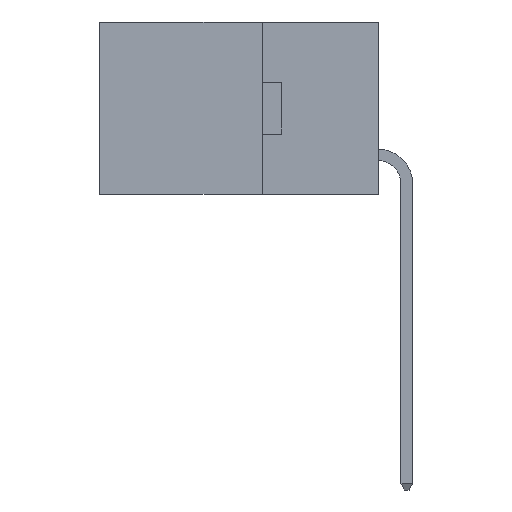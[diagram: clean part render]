
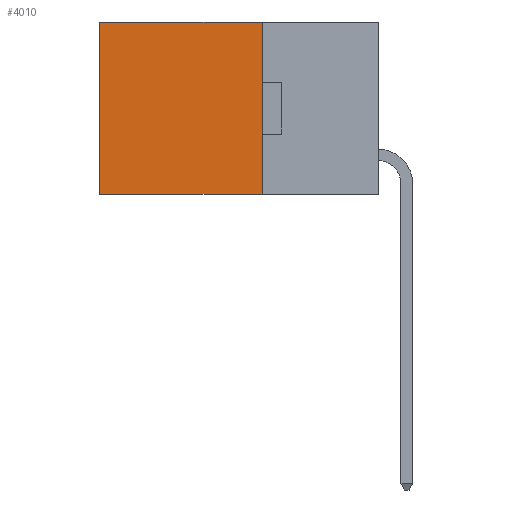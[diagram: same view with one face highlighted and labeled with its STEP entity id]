
A CAD part, left-side view. The second image highlights one B-rep face of the part: STEP entity #4010.
In plain terms, the highlighted planar face has unit normal (-1, 0, 0).
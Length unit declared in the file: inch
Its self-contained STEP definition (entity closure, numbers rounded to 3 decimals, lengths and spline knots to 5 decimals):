
#916 = CARTESIAN_POINT ( 'NONE',  ( 0.2615, 0.25, -0.37 ) ) ;
#2345 = LINE ( 'NONE', #15793, #16446 ) ;
#2472 = EDGE_CURVE ( 'NONE', #17665, #14523, #2345, .T. ) ;
#2713 = EDGE_CURVE ( 'NONE', #25090, #12654, #26334, .T. ) ;
#4010 = ADVANCED_FACE ( 'NONE', ( #21203 ), #24283, .F. ) ;
#4569 = CARTESIAN_POINT ( 'NONE',  ( 0.2615, 0.6, 0. ) ) ;
#4777 = EDGE_LOOP ( 'NONE', ( #15254, #18276, #24194, #24039 ) ) ;
#4930 = VECTOR ( 'NONE', #5220, 39.37008 ) ;
#5220 = DIRECTION ( 'NONE',  ( 0., 0., -1. ) ) ;
#6116 = CARTESIAN_POINT ( 'NONE',  ( 0.2615, 0.25, 0. ) ) ;
#8182 = CARTESIAN_POINT ( 'NONE',  ( 0.2615, 0.6, -0.37 ) ) ;
#8214 = EDGE_CURVE ( 'NONE', #17665, #25090, #16729, .T. ) ;
#10292 = DIRECTION ( 'NONE',  ( 0., 0., -1. ) ) ;
#12654 = VERTEX_POINT ( 'NONE', #14967 ) ;
#12839 = DIRECTION ( 'NONE',  ( 0., 1., 0. ) ) ;
#13164 = LINE ( 'NONE', #8182, #23462 ) ;
#14523 = VERTEX_POINT ( 'NONE', #4569 ) ;
#14967 = CARTESIAN_POINT ( 'NONE',  ( 0.2615, 0.6, -0.37 ) ) ;
#15254 = ORIENTED_EDGE ( 'NONE', *, *, #17017, .T. ) ;
#15793 = CARTESIAN_POINT ( 'NONE',  ( 0.2615, 0.25, 0. ) ) ;
#16446 = VECTOR ( 'NONE', #19413, 39.37008 ) ;
#16729 = LINE ( 'NONE', #23851, #4930 ) ;
#17017 = EDGE_CURVE ( 'NONE', #14523, #12654, #13164, .T. ) ;
#17665 = VERTEX_POINT ( 'NONE', #6116 ) ;
#18276 = ORIENTED_EDGE ( 'NONE', *, *, #2713, .F. ) ;
#19413 = DIRECTION ( 'NONE',  ( 0., 1., 0. ) ) ;
#20284 = AXIS2_PLACEMENT_3D ( 'NONE', #25554, #24576, #25626 ) ;
#20911 = VECTOR ( 'NONE', #12839, 39.37008 ) ;
#21203 = FACE_OUTER_BOUND ( 'NONE', #4777, .T. ) ;
#23462 = VECTOR ( 'NONE', #10292, 39.37008 ) ;
#23851 = CARTESIAN_POINT ( 'NONE',  ( 0.2615, 0.25, -0.37 ) ) ;
#24039 = ORIENTED_EDGE ( 'NONE', *, *, #2472, .T. ) ;
#24194 = ORIENTED_EDGE ( 'NONE', *, *, #8214, .F. ) ;
#24283 = PLANE ( 'NONE',  #20284 ) ;
#24576 = DIRECTION ( 'NONE',  ( 1., 0., 0. ) ) ;
#25090 = VERTEX_POINT ( 'NONE', #25920 ) ;
#25554 = CARTESIAN_POINT ( 'NONE',  ( 0.2615, 0.25, -0.37 ) ) ;
#25626 = DIRECTION ( 'NONE',  ( 0., 0., -1. ) ) ;
#25920 = CARTESIAN_POINT ( 'NONE',  ( 0.2615, 0.25, -0.37 ) ) ;
#26334 = LINE ( 'NONE', #916, #20911 ) ;
